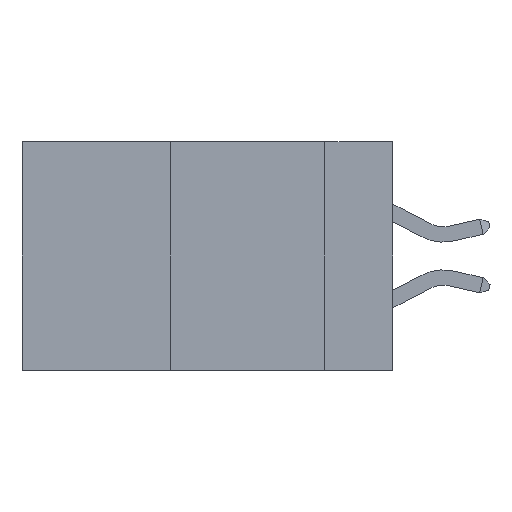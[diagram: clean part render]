
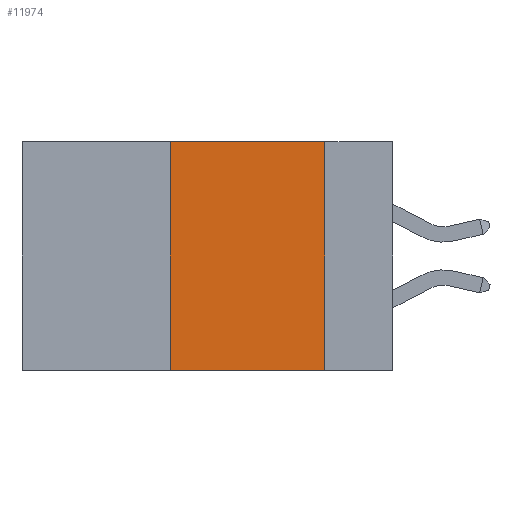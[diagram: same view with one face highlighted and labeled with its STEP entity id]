
A CAD part, left-side view. The second image highlights one B-rep face of the part: STEP entity #11974.
In plain terms, the highlighted planar face has unit normal (-1, 0, 0).
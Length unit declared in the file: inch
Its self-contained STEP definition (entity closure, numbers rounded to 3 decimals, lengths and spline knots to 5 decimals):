
#149 = DIRECTION ( 'NONE',  ( 0., 0., -1. ) ) ;
#341 = ORIENTED_EDGE ( 'NONE', *, *, #21987, .F. ) ;
#5540 = DIRECTION ( 'NONE',  ( 1., 0., 0. ) ) ;
#6464 = VECTOR ( 'NONE', #24388, 39.37008 ) ;
#7217 = EDGE_CURVE ( 'NONE', #18670, #25089, #9009, .T. ) ;
#8398 = VERTEX_POINT ( 'NONE', #20204 ) ;
#8400 = ORIENTED_EDGE ( 'NONE', *, *, #7217, .F. ) ;
#8959 = VERTEX_POINT ( 'NONE', #26557 ) ;
#9009 = LINE ( 'NONE', #29549, #28045 ) ;
#9194 = VECTOR ( 'NONE', #32047, 39.37008 ) ;
#9949 = CARTESIAN_POINT ( 'NONE',  ( 0., 0.36, 0. ) ) ;
#11974 = ADVANCED_FACE ( 'NONE', ( #32561 ), #20560, .F. ) ;
#12812 = CARTESIAN_POINT ( 'NONE',  ( 0., 0.11, 0. ) ) ;
#12876 = LINE ( 'NONE', #30831, #34137 ) ;
#13316 = DIRECTION ( 'NONE',  ( 0., -1., 0. ) ) ;
#14451 = EDGE_LOOP ( 'NONE', ( #23574, #8400, #341, #16516 ) ) ;
#16516 = ORIENTED_EDGE ( 'NONE', *, *, #16578, .T. ) ;
#16578 = EDGE_CURVE ( 'NONE', #8959, #8398, #18306, .T. ) ;
#18118 = LINE ( 'NONE', #12812, #9194 ) ;
#18306 = LINE ( 'NONE', #29650, #6464 ) ;
#18670 = VERTEX_POINT ( 'NONE', #9949 ) ;
#19754 = EDGE_CURVE ( 'NONE', #25089, #8398, #18118, .T. ) ;
#20204 = CARTESIAN_POINT ( 'NONE',  ( 0., 0.11, -0.37 ) ) ;
#20537 = CARTESIAN_POINT ( 'NONE',  ( 0., 0.11, 0. ) ) ;
#20560 = PLANE ( 'NONE',  #28057 ) ;
#21064 = DIRECTION ( 'NONE',  ( 0., 0., 1. ) ) ;
#21987 = EDGE_CURVE ( 'NONE', #8959, #18670, #12876, .T. ) ;
#23574 = ORIENTED_EDGE ( 'NONE', *, *, #19754, .F. ) ;
#24388 = DIRECTION ( 'NONE',  ( 0., -1., 0. ) ) ;
#25089 = VERTEX_POINT ( 'NONE', #20537 ) ;
#26557 = CARTESIAN_POINT ( 'NONE',  ( 0., 0.36, -0.37 ) ) ;
#28045 = VECTOR ( 'NONE', #13316, 39.37008 ) ;
#28057 = AXIS2_PLACEMENT_3D ( 'NONE', #29685, #5540, #149 ) ;
#29549 = CARTESIAN_POINT ( 'NONE',  ( 0., 0.6, 0. ) ) ;
#29650 = CARTESIAN_POINT ( 'NONE',  ( 0., 0.6, -0.37 ) ) ;
#29685 = CARTESIAN_POINT ( 'NONE',  ( 0., 0.6, 0. ) ) ;
#30831 = CARTESIAN_POINT ( 'NONE',  ( 0., 0.36, 0. ) ) ;
#32047 = DIRECTION ( 'NONE',  ( 0., 0., -1. ) ) ;
#32561 = FACE_OUTER_BOUND ( 'NONE', #14451, .T. ) ;
#34137 = VECTOR ( 'NONE', #21064, 39.37008 ) ;
